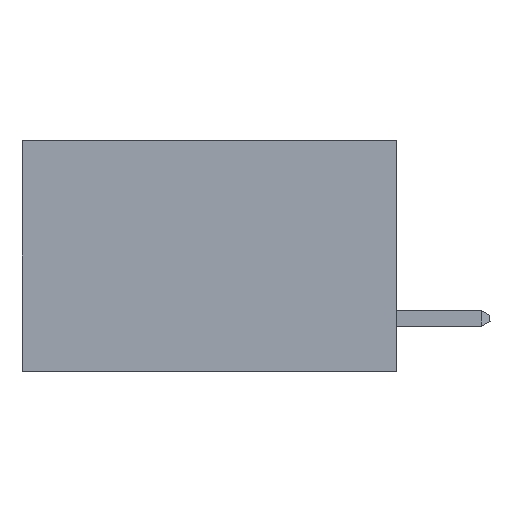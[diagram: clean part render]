
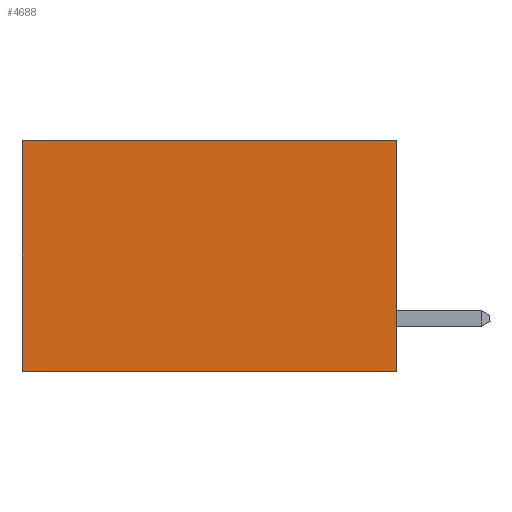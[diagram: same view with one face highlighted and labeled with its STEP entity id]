
A CAD part, left-side view. The second image highlights one B-rep face of the part: STEP entity #4688.
In plain terms, the highlighted planar face has unit normal (-1, 0, 0).
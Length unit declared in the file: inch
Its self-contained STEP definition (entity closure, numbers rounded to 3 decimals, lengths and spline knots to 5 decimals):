
#619 = VECTOR ( 'NONE', #1132, 39.37008 ) ;
#1132 = DIRECTION ( 'NONE',  ( 0., 0., -1. ) ) ;
#1719 = EDGE_CURVE ( 'NONE', #13201, #7986, #9822, .T. ) ;
#1749 = EDGE_CURVE ( 'NONE', #17103, #7986, #19266, .T. ) ;
#2207 = EDGE_CURVE ( 'NONE', #6085, #17103, #5701, .T. ) ;
#2591 = PLANE ( 'NONE',  #7954 ) ;
#4127 = ORIENTED_EDGE ( 'NONE', *, *, #7365, .T. ) ;
#4477 = CARTESIAN_POINT ( 'NONE',  ( 0.298, 0., -0.37 ) ) ;
#4688 = ADVANCED_FACE ( 'NONE', ( #20645 ), #2591, .F. ) ;
#5701 = LINE ( 'NONE', #21140, #11590 ) ;
#6035 = ORIENTED_EDGE ( 'NONE', *, *, #1749, .F. ) ;
#6085 = VERTEX_POINT ( 'NONE', #18471 ) ;
#7365 = EDGE_CURVE ( 'NONE', #6085, #13201, #9200, .T. ) ;
#7954 = AXIS2_PLACEMENT_3D ( 'NONE', #9189, #12472, #13967 ) ;
#7986 = VERTEX_POINT ( 'NONE', #21147 ) ;
#8214 = CARTESIAN_POINT ( 'NONE',  ( 0.298, 0., -0.37 ) ) ;
#9189 = CARTESIAN_POINT ( 'NONE',  ( 0.298, 0., 0. ) ) ;
#9200 = LINE ( 'NONE', #15979, #12777 ) ;
#9273 = DIRECTION ( 'NONE',  ( 0., 1., 0. ) ) ;
#9665 = DIRECTION ( 'NONE',  ( 0., 0., -1. ) ) ;
#9822 = LINE ( 'NONE', #19215, #619 ) ;
#11538 = ORIENTED_EDGE ( 'NONE', *, *, #2207, .F. ) ;
#11590 = VECTOR ( 'NONE', #9665, 39.37008 ) ;
#12123 = VECTOR ( 'NONE', #9273, 39.37008 ) ;
#12472 = DIRECTION ( 'NONE',  ( 1., 0., 0. ) ) ;
#12777 = VECTOR ( 'NONE', #20905, 39.37008 ) ;
#13201 = VERTEX_POINT ( 'NONE', #15541 ) ;
#13967 = DIRECTION ( 'NONE',  ( 0., 0., -1. ) ) ;
#15541 = CARTESIAN_POINT ( 'NONE',  ( 0.298, 0.6, 0. ) ) ;
#15979 = CARTESIAN_POINT ( 'NONE',  ( 0.298, 0., 0. ) ) ;
#16525 = ORIENTED_EDGE ( 'NONE', *, *, #1719, .T. ) ;
#17103 = VERTEX_POINT ( 'NONE', #4477 ) ;
#17532 = EDGE_LOOP ( 'NONE', ( #16525, #6035, #11538, #4127 ) ) ;
#18471 = CARTESIAN_POINT ( 'NONE',  ( 0.298, 0., 0. ) ) ;
#19215 = CARTESIAN_POINT ( 'NONE',  ( 0.298, 0.6, 0. ) ) ;
#19266 = LINE ( 'NONE', #8214, #12123 ) ;
#20645 = FACE_OUTER_BOUND ( 'NONE', #17532, .T. ) ;
#20905 = DIRECTION ( 'NONE',  ( 0., 1., 0. ) ) ;
#21140 = CARTESIAN_POINT ( 'NONE',  ( 0.298, 0., 0. ) ) ;
#21147 = CARTESIAN_POINT ( 'NONE',  ( 0.298, 0.6, -0.37 ) ) ;
